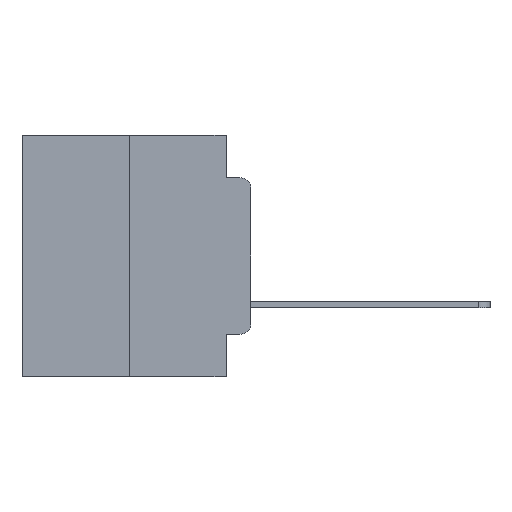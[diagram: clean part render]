
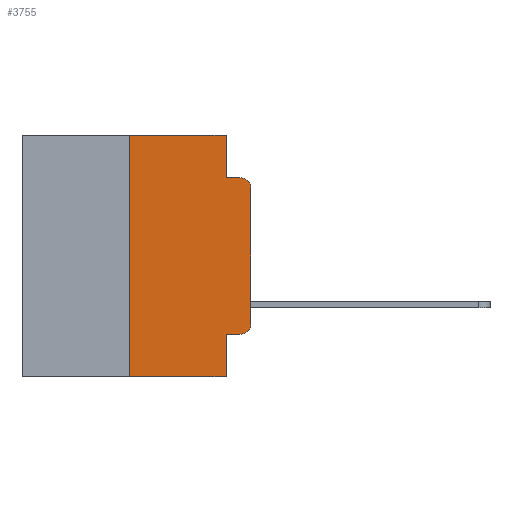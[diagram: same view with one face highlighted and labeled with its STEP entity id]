
A CAD part, left-side view. The second image highlights one B-rep face of the part: STEP entity #3755.
In plain terms, the highlighted planar face has unit normal (-1, 0, 0).
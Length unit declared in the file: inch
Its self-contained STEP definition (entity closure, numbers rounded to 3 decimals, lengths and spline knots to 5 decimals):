
#120 = CARTESIAN_POINT ( 'NONE',  ( 0., 0.02, -0.3915 ) ) ;
#271 = VERTEX_POINT ( 'NONE', #18910 ) ;
#1060 = ORIENTED_EDGE ( 'NONE', *, *, #11326, .T. ) ;
#2045 = VECTOR ( 'NONE', #14509, 39.37008 ) ;
#2326 = VERTEX_POINT ( 'NONE', #22798 ) ;
#2376 = VECTOR ( 'NONE', #7035, 39.37008 ) ;
#2424 = EDGE_CURVE ( 'NONE', #271, #15388, #4334, .T. ) ;
#2793 = EDGE_CURVE ( 'NONE', #8520, #271, #23655, .T. ) ;
#2907 = ORIENTED_EDGE ( 'NONE', *, *, #2793, .F. ) ;
#3339 = DIRECTION ( 'NONE',  ( 1., 0., 0. ) ) ;
#3755 = ADVANCED_FACE ( 'NONE', ( #16109 ), #22236, .F. ) ;
#3888 = VERTEX_POINT ( 'NONE', #16087 ) ;
#4156 = CARTESIAN_POINT ( 'NONE',  ( 0., 0.02, -0.1085 ) ) ;
#4334 = LINE ( 'NONE', #16975, #2045 ) ;
#4568 = EDGE_LOOP ( 'NONE', ( #1060, #20277, #18284, #25214, #2907, #12144, #8304, #12325, #5875, #16225 ) ) ;
#5136 = CARTESIAN_POINT ( 'NONE',  ( 0., 0.25, 0. ) ) ;
#5875 = ORIENTED_EDGE ( 'NONE', *, *, #12320, .T. ) ;
#6233 = VERTEX_POINT ( 'NONE', #11307 ) ;
#6259 = LINE ( 'NONE', #12770, #11151 ) ;
#6290 = DIRECTION ( 'NONE',  ( 0., 0., -1. ) ) ;
#7035 = DIRECTION ( 'NONE',  ( 0., -1., 0. ) ) ;
#7688 = AXIS2_PLACEMENT_3D ( 'NONE', #11747, #3339, #17645 ) ;
#8150 = AXIS2_PLACEMENT_3D ( 'NONE', #120, #8561, #23231 ) ;
#8304 = ORIENTED_EDGE ( 'NONE', *, *, #14326, .T. ) ;
#8397 = AXIS2_PLACEMENT_3D ( 'NONE', #4156, #12492, #23059 ) ;
#8520 = VERTEX_POINT ( 'NONE', #5136 ) ;
#8561 = DIRECTION ( 'NONE',  ( -1., 0., 0. ) ) ;
#9254 = CARTESIAN_POINT ( 'NONE',  ( 0., 0., 0. ) ) ;
#9275 = VECTOR ( 'NONE', #19363, 39.37008 ) ;
#9284 = VERTEX_POINT ( 'NONE', #11549 ) ;
#9860 = CARTESIAN_POINT ( 'NONE',  ( 0., 0.02, -0.4115 ) ) ;
#10757 = EDGE_CURVE ( 'NONE', #18740, #8520, #19127, .T. ) ;
#11151 = VECTOR ( 'NONE', #6290, 39.37008 ) ;
#11307 = CARTESIAN_POINT ( 'NONE',  ( 0., 0., -0.1085 ) ) ;
#11326 = EDGE_CURVE ( 'NONE', #3888, #6233, #13134, .T. ) ;
#11375 = VERTEX_POINT ( 'NONE', #22061 ) ;
#11445 = CIRCLE ( 'NONE', #8150, 0.02 ) ;
#11549 = CARTESIAN_POINT ( 'NONE',  ( 0., 0.02, -0.0885 ) ) ;
#11747 = CARTESIAN_POINT ( 'NONE',  ( 0., 0.473, 0. ) ) ;
#11802 = CARTESIAN_POINT ( 'NONE',  ( 0., 0.473, 0. ) ) ;
#12144 = ORIENTED_EDGE ( 'NONE', *, *, #10757, .F. ) ;
#12204 = EDGE_CURVE ( 'NONE', #14048, #3888, #11445, .T. ) ;
#12320 = EDGE_CURVE ( 'NONE', #11375, #14048, #23587, .T. ) ;
#12325 = ORIENTED_EDGE ( 'NONE', *, *, #22523, .F. ) ;
#12492 = DIRECTION ( 'NONE',  ( -1., 0., 0. ) ) ;
#12642 = CARTESIAN_POINT ( 'NONE',  ( 0., 0.25, 0. ) ) ;
#12770 = CARTESIAN_POINT ( 'NONE',  ( 0., 0.051, 0. ) ) ;
#13134 = LINE ( 'NONE', #9254, #24303 ) ;
#13584 = EDGE_CURVE ( 'NONE', #15388, #9284, #22128, .T. ) ;
#14048 = VERTEX_POINT ( 'NONE', #9860 ) ;
#14326 = EDGE_CURVE ( 'NONE', #18740, #2326, #17844, .T. ) ;
#14509 = DIRECTION ( 'NONE',  ( 0., 0., -1. ) ) ;
#15388 = VERTEX_POINT ( 'NONE', #17243 ) ;
#16087 = CARTESIAN_POINT ( 'NONE',  ( 0., 0., -0.3915 ) ) ;
#16109 = FACE_OUTER_BOUND ( 'NONE', #4568, .T. ) ;
#16225 = ORIENTED_EDGE ( 'NONE', *, *, #12204, .T. ) ;
#16465 = DIRECTION ( 'NONE',  ( 0., -1., 0. ) ) ;
#16615 = CARTESIAN_POINT ( 'NONE',  ( 0., 0.25, -0.5 ) ) ;
#16975 = CARTESIAN_POINT ( 'NONE',  ( 0., 0.051, 0. ) ) ;
#17243 = CARTESIAN_POINT ( 'NONE',  ( 0., 0.051, -0.0885 ) ) ;
#17645 = DIRECTION ( 'NONE',  ( 0., 0., -1. ) ) ;
#17844 = LINE ( 'NONE', #23789, #2376 ) ;
#17890 = DIRECTION ( 'NONE',  ( 0., -1., 0. ) ) ;
#18053 = VECTOR ( 'NONE', #16465, 39.37008 ) ;
#18284 = ORIENTED_EDGE ( 'NONE', *, *, #13584, .F. ) ;
#18740 = VERTEX_POINT ( 'NONE', #16615 ) ;
#18783 = CARTESIAN_POINT ( 'NONE',  ( 0., 0.051, -0.4115 ) ) ;
#18910 = CARTESIAN_POINT ( 'NONE',  ( 0., 0.051, 0. ) ) ;
#19127 = LINE ( 'NONE', #12642, #9275 ) ;
#19363 = DIRECTION ( 'NONE',  ( 0., 0., 1. ) ) ;
#19852 = VECTOR ( 'NONE', #25385, 39.37008 ) ;
#19989 = DIRECTION ( 'NONE',  ( 0., 0., 1. ) ) ;
#20277 = ORIENTED_EDGE ( 'NONE', *, *, #21159, .T. ) ;
#21159 = EDGE_CURVE ( 'NONE', #6233, #9284, #21724, .T. ) ;
#21361 = CARTESIAN_POINT ( 'NONE',  ( 0., 0.051, -0.0885 ) ) ;
#21724 = CIRCLE ( 'NONE', #8397, 0.02 ) ;
#22061 = CARTESIAN_POINT ( 'NONE',  ( 0., 0.051, -0.4115 ) ) ;
#22128 = LINE ( 'NONE', #21361, #19852 ) ;
#22236 = PLANE ( 'NONE',  #7688 ) ;
#22523 = EDGE_CURVE ( 'NONE', #11375, #2326, #6259, .T. ) ;
#22798 = CARTESIAN_POINT ( 'NONE',  ( 0., 0.051, -0.5 ) ) ;
#23059 = DIRECTION ( 'NONE',  ( 0., 0., -1. ) ) ;
#23231 = DIRECTION ( 'NONE',  ( 0., 0., -1. ) ) ;
#23587 = LINE ( 'NONE', #18783, #18053 ) ;
#23655 = LINE ( 'NONE', #11802, #24657 ) ;
#23789 = CARTESIAN_POINT ( 'NONE',  ( 0., 0.473, -0.5 ) ) ;
#24303 = VECTOR ( 'NONE', #19989, 39.37008 ) ;
#24657 = VECTOR ( 'NONE', #17890, 39.37008 ) ;
#25214 = ORIENTED_EDGE ( 'NONE', *, *, #2424, .F. ) ;
#25385 = DIRECTION ( 'NONE',  ( 0., -1., 0. ) ) ;
